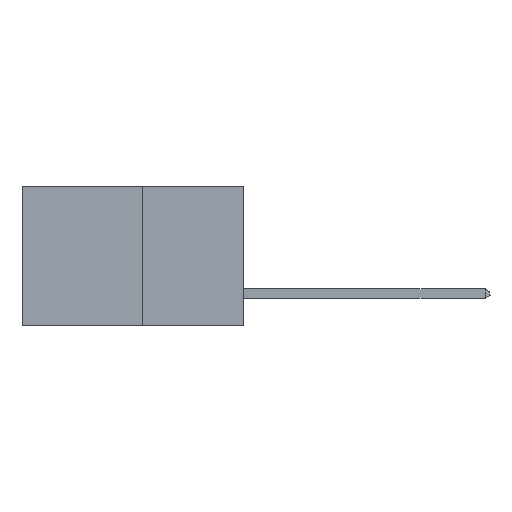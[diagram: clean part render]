
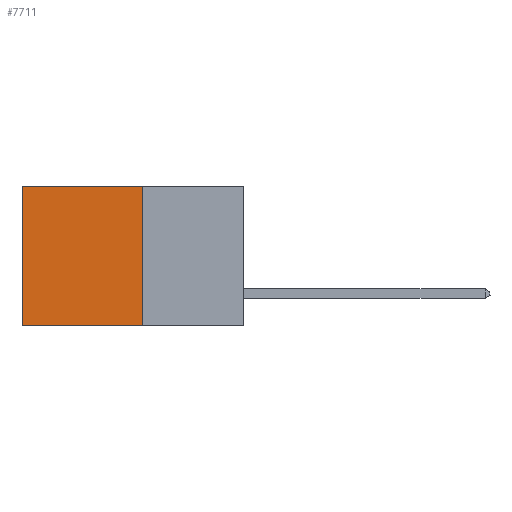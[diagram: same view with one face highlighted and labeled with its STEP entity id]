
A CAD part, left-side view. The second image highlights one B-rep face of the part: STEP entity #7711.
In plain terms, the highlighted planar face has unit normal (-1, 0, 0).
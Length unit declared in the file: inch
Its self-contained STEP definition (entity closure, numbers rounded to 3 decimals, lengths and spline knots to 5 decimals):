
#466 = CARTESIAN_POINT ( 'NONE',  ( 0.277, 0.27, -0.37 ) ) ;
#555 = AXIS2_PLACEMENT_3D ( 'NONE', #2208, #2211, #2124 ) ;
#982 = LINE ( 'NONE', #7585, #5346 ) ;
#1638 = FACE_OUTER_BOUND ( 'NONE', #4955, .T. ) ;
#1768 = DIRECTION ( 'NONE',  ( 0., 1., 0. ) ) ;
#2124 = DIRECTION ( 'NONE',  ( 0., 0., -1. ) ) ;
#2208 = CARTESIAN_POINT ( 'NONE',  ( 0.277, 0.27, -0.37 ) ) ;
#2211 = DIRECTION ( 'NONE',  ( 1., 0., 0. ) ) ;
#2672 = ORIENTED_EDGE ( 'NONE', *, *, #11470, .F. ) ;
#2813 = CARTESIAN_POINT ( 'NONE',  ( 0.277, 0.27, -0.37 ) ) ;
#3048 = ORIENTED_EDGE ( 'NONE', *, *, #7324, .T. ) ;
#3870 = DIRECTION ( 'NONE',  ( 0., 1., 0. ) ) ;
#4031 = DIRECTION ( 'NONE',  ( 0., 0., -1. ) ) ;
#4704 = CARTESIAN_POINT ( 'NONE',  ( 0.277, 0.59, 0. ) ) ;
#4747 = LINE ( 'NONE', #13282, #10789 ) ;
#4955 = EDGE_LOOP ( 'NONE', ( #5546, #2672, #14740, #3048 ) ) ;
#5346 = VECTOR ( 'NONE', #8699, 39.37008 ) ;
#5546 = ORIENTED_EDGE ( 'NONE', *, *, #11322, .T. ) ;
#6263 = CARTESIAN_POINT ( 'NONE',  ( 0.277, 0.27, 0. ) ) ;
#6574 = VERTEX_POINT ( 'NONE', #466 ) ;
#7324 = EDGE_CURVE ( 'NONE', #11476, #11097, #8788, .T. ) ;
#7585 = CARTESIAN_POINT ( 'NONE',  ( 0.277, 0.59, -0.37 ) ) ;
#7711 = ADVANCED_FACE ( 'NONE', ( #1638 ), #14040, .F. ) ;
#8699 = DIRECTION ( 'NONE',  ( 0., 0., -1. ) ) ;
#8788 = LINE ( 'NONE', #6263, #13855 ) ;
#9614 = CARTESIAN_POINT ( 'NONE',  ( 0.277, 0.59, -0.37 ) ) ;
#10789 = VECTOR ( 'NONE', #1768, 39.37008 ) ;
#11097 = VERTEX_POINT ( 'NONE', #4704 ) ;
#11322 = EDGE_CURVE ( 'NONE', #11097, #11819, #982, .T. ) ;
#11470 = EDGE_CURVE ( 'NONE', #6574, #11819, #4747, .T. ) ;
#11476 = VERTEX_POINT ( 'NONE', #12232 ) ;
#11819 = VERTEX_POINT ( 'NONE', #9614 ) ;
#12211 = EDGE_CURVE ( 'NONE', #11476, #6574, #12845, .T. ) ;
#12232 = CARTESIAN_POINT ( 'NONE',  ( 0.277, 0.27, 0. ) ) ;
#12495 = VECTOR ( 'NONE', #4031, 39.37008 ) ;
#12845 = LINE ( 'NONE', #2813, #12495 ) ;
#13282 = CARTESIAN_POINT ( 'NONE',  ( 0.277, 0.27, -0.37 ) ) ;
#13855 = VECTOR ( 'NONE', #3870, 39.37008 ) ;
#14040 = PLANE ( 'NONE',  #555 ) ;
#14740 = ORIENTED_EDGE ( 'NONE', *, *, #12211, .F. ) ;
